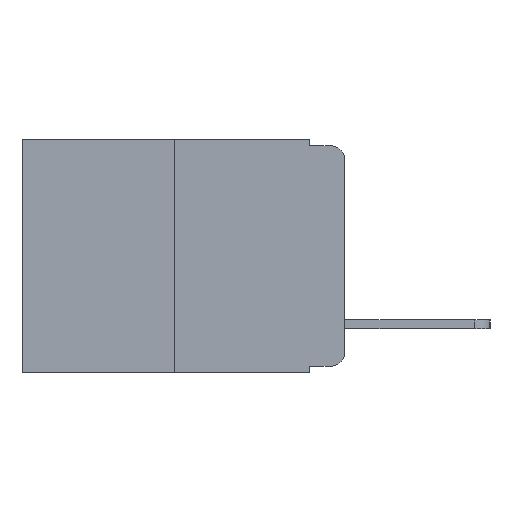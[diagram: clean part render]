
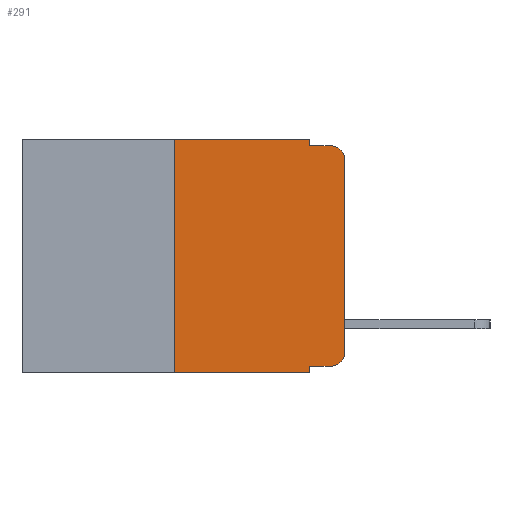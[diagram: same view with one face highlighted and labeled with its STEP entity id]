
A CAD part, left-side view. The second image highlights one B-rep face of the part: STEP entity #291.
In plain terms, the highlighted planar face has unit normal (-1, 0, 0).
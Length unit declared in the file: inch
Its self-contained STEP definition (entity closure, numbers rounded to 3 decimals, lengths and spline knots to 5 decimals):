
#203 = DIRECTION ( 'NONE',  ( 0., 0., -1. ) ) ;
#291 = ADVANCED_FACE ( 'NONE', ( #2894 ), #9739, .F. ) ;
#390 = VERTEX_POINT ( 'NONE', #11596 ) ;
#538 = CARTESIAN_POINT ( 'NONE',  ( 0., 0.051, -0.01 ) ) ;
#657 = ORIENTED_EDGE ( 'NONE', *, *, #7576, .T. ) ;
#1273 = AXIS2_PLACEMENT_3D ( 'NONE', #4409, #11722, #5573 ) ;
#1971 = VECTOR ( 'NONE', #2063, 39.37008 ) ;
#2063 = DIRECTION ( 'NONE',  ( 0., 0., -1. ) ) ;
#2372 = VECTOR ( 'NONE', #7682, 39.37008 ) ;
#2469 = VECTOR ( 'NONE', #11768, 39.37008 ) ;
#2741 = CIRCLE ( 'NONE', #1273, 0.02 ) ;
#2894 = FACE_OUTER_BOUND ( 'NONE', #3830, .T. ) ;
#3145 = LINE ( 'NONE', #11191, #14247 ) ;
#3234 = ORIENTED_EDGE ( 'NONE', *, *, #7271, .F. ) ;
#3519 = VERTEX_POINT ( 'NONE', #5917 ) ;
#3829 = EDGE_CURVE ( 'NONE', #7171, #14178, #13724, .T. ) ;
#3830 = EDGE_LOOP ( 'NONE', ( #5986, #4172, #4928, #3234, #10523, #12682, #4961, #12824, #8217, #657 ) ) ;
#4172 = ORIENTED_EDGE ( 'NONE', *, *, #7269, .T. ) ;
#4409 = CARTESIAN_POINT ( 'NONE',  ( 0., 0.02, -0.03 ) ) ;
#4622 = CARTESIAN_POINT ( 'NONE',  ( 0., 0.051, -0.333 ) ) ;
#4644 = DIRECTION ( 'NONE',  ( 1., 0., 0. ) ) ;
#4699 = CARTESIAN_POINT ( 'NONE',  ( 0., 0.051, -0.343 ) ) ;
#4928 = ORIENTED_EDGE ( 'NONE', *, *, #7270, .F. ) ;
#4961 = ORIENTED_EDGE ( 'NONE', *, *, #6902, .T. ) ;
#5192 = LINE ( 'NONE', #10748, #1971 ) ;
#5198 = CARTESIAN_POINT ( 'NONE',  ( 0., 0.051, 0. ) ) ;
#5573 = DIRECTION ( 'NONE',  ( 0., 0., -1. ) ) ;
#5674 = CARTESIAN_POINT ( 'NONE',  ( 0., 0.051, -0.333 ) ) ;
#5767 = DIRECTION ( 'NONE',  ( 0., -1., 0. ) ) ;
#5917 = CARTESIAN_POINT ( 'NONE',  ( 0., 0.25, -0.343 ) ) ;
#5986 = ORIENTED_EDGE ( 'NONE', *, *, #7250, .T. ) ;
#6095 = CARTESIAN_POINT ( 'NONE',  ( 0., 0.02, -0.333 ) ) ;
#6471 = VERTEX_POINT ( 'NONE', #9752 ) ;
#6532 = DIRECTION ( 'NONE',  ( 0., -1., 0. ) ) ;
#6578 = CARTESIAN_POINT ( 'NONE',  ( 0., 0.051, 0. ) ) ;
#6649 = AXIS2_PLACEMENT_3D ( 'NONE', #11384, #4644, #203 ) ;
#6902 = EDGE_CURVE ( 'NONE', #3519, #7467, #3145, .T. ) ;
#7014 = DIRECTION ( 'NONE',  ( -1., 0., 0. ) ) ;
#7171 = VERTEX_POINT ( 'NONE', #10568 ) ;
#7250 = EDGE_CURVE ( 'NONE', #8456, #6471, #8947, .T. ) ;
#7269 = EDGE_CURVE ( 'NONE', #6471, #10840, #2741, .T. ) ;
#7270 = EDGE_CURVE ( 'NONE', #390, #10840, #13647, .T. ) ;
#7271 = EDGE_CURVE ( 'NONE', #14178, #390, #11053, .T. ) ;
#7290 = EDGE_CURVE ( 'NONE', #3519, #7171, #13348, .T. ) ;
#7291 = EDGE_CURVE ( 'NONE', #8569, #7467, #5192, .T. ) ;
#7361 = EDGE_CURVE ( 'NONE', #8569, #9050, #9796, .T. ) ;
#7467 = VERTEX_POINT ( 'NONE', #4699 ) ;
#7576 = EDGE_CURVE ( 'NONE', #9050, #8456, #8936, .T. ) ;
#7682 = DIRECTION ( 'NONE',  ( 0., 0., -1. ) ) ;
#7734 = DIRECTION ( 'NONE',  ( 0., 0., 1. ) ) ;
#8217 = ORIENTED_EDGE ( 'NONE', *, *, #7361, .T. ) ;
#8323 = VECTOR ( 'NONE', #6532, 39.37008 ) ;
#8456 = VERTEX_POINT ( 'NONE', #12721 ) ;
#8569 = VERTEX_POINT ( 'NONE', #5674 ) ;
#8936 = CIRCLE ( 'NONE', #10951, 0.02 ) ;
#8947 = LINE ( 'NONE', #10700, #13945 ) ;
#9050 = VERTEX_POINT ( 'NONE', #6095 ) ;
#9739 = PLANE ( 'NONE',  #6649 ) ;
#9752 = CARTESIAN_POINT ( 'NONE',  ( 0., 0., -0.03 ) ) ;
#9796 = LINE ( 'NONE', #4622, #12118 ) ;
#10489 = CARTESIAN_POINT ( 'NONE',  ( 0., 0.02, -0.01 ) ) ;
#10523 = ORIENTED_EDGE ( 'NONE', *, *, #3829, .F. ) ;
#10568 = CARTESIAN_POINT ( 'NONE',  ( 0., 0.25, 0. ) ) ;
#10700 = CARTESIAN_POINT ( 'NONE',  ( 0., 0., 0. ) ) ;
#10748 = CARTESIAN_POINT ( 'NONE',  ( 0., 0.051, 0. ) ) ;
#10757 = CARTESIAN_POINT ( 'NONE',  ( 0., 0.473, 0. ) ) ;
#10840 = VERTEX_POINT ( 'NONE', #10489 ) ;
#10951 = AXIS2_PLACEMENT_3D ( 'NONE', #13124, #7014, #14062 ) ;
#11053 = LINE ( 'NONE', #6578, #2372 ) ;
#11191 = CARTESIAN_POINT ( 'NONE',  ( 0., 0.473, -0.343 ) ) ;
#11384 = CARTESIAN_POINT ( 'NONE',  ( 0., 0.473, 0. ) ) ;
#11596 = CARTESIAN_POINT ( 'NONE',  ( 0., 0.051, -0.01 ) ) ;
#11680 = DIRECTION ( 'NONE',  ( 0., 0., 1. ) ) ;
#11722 = DIRECTION ( 'NONE',  ( -1., 0., 0. ) ) ;
#11768 = DIRECTION ( 'NONE',  ( 0., -1., 0. ) ) ;
#12118 = VECTOR ( 'NONE', #5767, 39.37008 ) ;
#12682 = ORIENTED_EDGE ( 'NONE', *, *, #7290, .F. ) ;
#12721 = CARTESIAN_POINT ( 'NONE',  ( 0., 0., -0.313 ) ) ;
#12764 = CARTESIAN_POINT ( 'NONE',  ( 0., 0.25, 0. ) ) ;
#12824 = ORIENTED_EDGE ( 'NONE', *, *, #7291, .F. ) ;
#13059 = VECTOR ( 'NONE', #7734, 39.37008 ) ;
#13124 = CARTESIAN_POINT ( 'NONE',  ( 0., 0.02, -0.313 ) ) ;
#13126 = DIRECTION ( 'NONE',  ( 0., -1., 0. ) ) ;
#13348 = LINE ( 'NONE', #12764, #13059 ) ;
#13647 = LINE ( 'NONE', #538, #8323 ) ;
#13724 = LINE ( 'NONE', #10757, #2469 ) ;
#13945 = VECTOR ( 'NONE', #11680, 39.37008 ) ;
#14062 = DIRECTION ( 'NONE',  ( 0., 0., -1. ) ) ;
#14178 = VERTEX_POINT ( 'NONE', #5198 ) ;
#14247 = VECTOR ( 'NONE', #13126, 39.37008 ) ;
